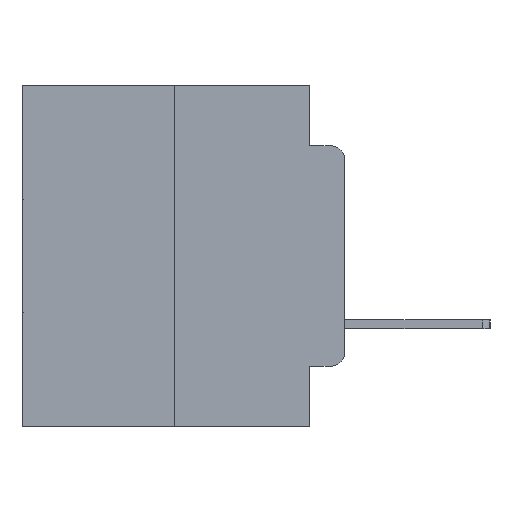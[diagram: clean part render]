
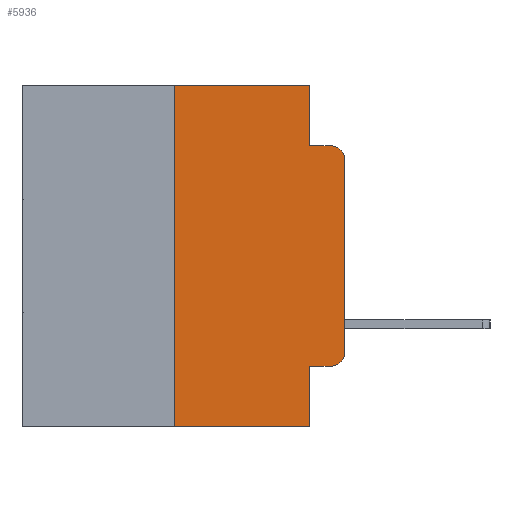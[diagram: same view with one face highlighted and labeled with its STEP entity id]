
A CAD part, left-side view. The second image highlights one B-rep face of the part: STEP entity #5936.
In plain terms, the highlighted planar face has unit normal (-1, 0, 0).
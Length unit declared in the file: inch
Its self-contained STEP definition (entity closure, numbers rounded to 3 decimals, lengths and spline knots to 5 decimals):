
#39 = DIRECTION ( 'NONE',  ( 0., -1., 0. ) ) ;
#232 = CARTESIAN_POINT ( 'NONE',  ( 0., 0.02, -0.4115 ) ) ;
#286 = VECTOR ( 'NONE', #25031, 39.37008 ) ;
#444 = EDGE_CURVE ( 'NONE', #7552, #21658, #17296, .T. ) ;
#829 = VERTEX_POINT ( 'NONE', #16610 ) ;
#1479 = DIRECTION ( 'NONE',  ( 0., -1., 0. ) ) ;
#1516 = ORIENTED_EDGE ( 'NONE', *, *, #5882, .T. ) ;
#1777 = LINE ( 'NONE', #26739, #12896 ) ;
#1890 = ORIENTED_EDGE ( 'NONE', *, *, #24686, .T. ) ;
#2066 = CARTESIAN_POINT ( 'NONE',  ( 0., 0.02, -0.3915 ) ) ;
#2331 = DIRECTION ( 'NONE',  ( 0., -1., 0. ) ) ;
#2914 = ORIENTED_EDGE ( 'NONE', *, *, #16534, .F. ) ;
#3414 = ORIENTED_EDGE ( 'NONE', *, *, #444, .F. ) ;
#3684 = ORIENTED_EDGE ( 'NONE', *, *, #9267, .F. ) ;
#3862 = AXIS2_PLACEMENT_3D ( 'NONE', #11210, #25497, #13319 ) ;
#3930 = ORIENTED_EDGE ( 'NONE', *, *, #17087, .F. ) ;
#3967 = EDGE_CURVE ( 'NONE', #19862, #829, #14197, .T. ) ;
#4100 = ORIENTED_EDGE ( 'NONE', *, *, #17632, .T. ) ;
#4322 = DIRECTION ( 'NONE',  ( 0., 0., -1. ) ) ;
#4430 = ORIENTED_EDGE ( 'NONE', *, *, #6991, .F. ) ;
#4480 = CARTESIAN_POINT ( 'NONE',  ( 0., 0.051, -0.5 ) ) ;
#4484 = ORIENTED_EDGE ( 'NONE', *, *, #5492, .T. ) ;
#4517 = VERTEX_POINT ( 'NONE', #4480 ) ;
#4648 = ORIENTED_EDGE ( 'NONE', *, *, #3967, .T. ) ;
#5492 = EDGE_CURVE ( 'NONE', #26529, #19862, #8429, .T. ) ;
#5882 = EDGE_CURVE ( 'NONE', #829, #21941, #13429, .T. ) ;
#5936 = ADVANCED_FACE ( 'NONE', ( #17036 ), #15282, .F. ) ;
#5951 = LINE ( 'NONE', #19071, #22824 ) ;
#6254 = DIRECTION ( 'NONE',  ( 0., 0., 1. ) ) ;
#6708 = CARTESIAN_POINT ( 'NONE',  ( 0., 0.25, -0.5 ) ) ;
#6991 = EDGE_CURVE ( 'NONE', #26529, #4517, #25455, .T. ) ;
#7493 = CARTESIAN_POINT ( 'NONE',  ( 0., 0.25, 0. ) ) ;
#7552 = VERTEX_POINT ( 'NONE', #13449 ) ;
#8314 = VECTOR ( 'NONE', #17233, 39.37008 ) ;
#8429 = LINE ( 'NONE', #15481, #24329 ) ;
#8680 = CIRCLE ( 'NONE', #3862, 0.02 ) ;
#9267 = EDGE_CURVE ( 'NONE', #25586, #7552, #17662, .T. ) ;
#10751 = CARTESIAN_POINT ( 'NONE',  ( 0., 0.051, -0.4115 ) ) ;
#10934 = CARTESIAN_POINT ( 'NONE',  ( 0., 0.051, 0. ) ) ;
#11016 = AXIS2_PLACEMENT_3D ( 'NONE', #2066, #17320, #4322 ) ;
#11167 = DIRECTION ( 'NONE',  ( 0., 0., -1. ) ) ;
#11210 = CARTESIAN_POINT ( 'NONE',  ( 0., 0.02, -0.1085 ) ) ;
#11452 = LINE ( 'NONE', #23502, #20583 ) ;
#12809 = VECTOR ( 'NONE', #15016, 39.37008 ) ;
#12842 = CARTESIAN_POINT ( 'NONE',  ( 0., 0.473, 0. ) ) ;
#12896 = VECTOR ( 'NONE', #1479, 39.37008 ) ;
#13020 = CARTESIAN_POINT ( 'NONE',  ( 0., 0., 0. ) ) ;
#13319 = DIRECTION ( 'NONE',  ( 0., 0., -1. ) ) ;
#13429 = LINE ( 'NONE', #13020, #12809 ) ;
#13449 = CARTESIAN_POINT ( 'NONE',  ( 0., 0.051, 0. ) ) ;
#14048 = DIRECTION ( 'NONE',  ( 0., 0., -1. ) ) ;
#14197 = CIRCLE ( 'NONE', #11016, 0.02 ) ;
#14690 = CARTESIAN_POINT ( 'NONE',  ( 0., 0.051, -0.0885 ) ) ;
#15016 = DIRECTION ( 'NONE',  ( 0., 0., 1. ) ) ;
#15102 = AXIS2_PLACEMENT_3D ( 'NONE', #19458, #23497, #11167 ) ;
#15282 = PLANE ( 'NONE',  #15102 ) ;
#15481 = CARTESIAN_POINT ( 'NONE',  ( 0., 0.051, -0.4115 ) ) ;
#15972 = VECTOR ( 'NONE', #14048, 39.37008 ) ;
#16534 = EDGE_CURVE ( 'NONE', #21658, #18693, #1777, .T. ) ;
#16610 = CARTESIAN_POINT ( 'NONE',  ( 0., 0., -0.3915 ) ) ;
#16893 = CARTESIAN_POINT ( 'NONE',  ( 0., 0.02, -0.0885 ) ) ;
#17036 = FACE_OUTER_BOUND ( 'NONE', #22107, .T. ) ;
#17087 = EDGE_CURVE ( 'NONE', #18920, #25586, #5951, .T. ) ;
#17233 = DIRECTION ( 'NONE',  ( 0., 0., -1. ) ) ;
#17296 = LINE ( 'NONE', #23672, #15972 ) ;
#17320 = DIRECTION ( 'NONE',  ( -1., 0., 0. ) ) ;
#17632 = EDGE_CURVE ( 'NONE', #18920, #4517, #11452, .T. ) ;
#17662 = LINE ( 'NONE', #12842, #286 ) ;
#18693 = VERTEX_POINT ( 'NONE', #16893 ) ;
#18920 = VERTEX_POINT ( 'NONE', #6708 ) ;
#19071 = CARTESIAN_POINT ( 'NONE',  ( 0., 0.25, 0. ) ) ;
#19458 = CARTESIAN_POINT ( 'NONE',  ( 0., 0.473, 0. ) ) ;
#19862 = VERTEX_POINT ( 'NONE', #232 ) ;
#20583 = VECTOR ( 'NONE', #39, 39.37008 ) ;
#21658 = VERTEX_POINT ( 'NONE', #14690 ) ;
#21941 = VERTEX_POINT ( 'NONE', #25573 ) ;
#22107 = EDGE_LOOP ( 'NONE', ( #1516, #1890, #2914, #3414, #3684, #3930, #4100, #4430, #4484, #4648 ) ) ;
#22824 = VECTOR ( 'NONE', #6254, 39.37008 ) ;
#23497 = DIRECTION ( 'NONE',  ( 1., 0., 0. ) ) ;
#23502 = CARTESIAN_POINT ( 'NONE',  ( 0., 0.473, -0.5 ) ) ;
#23672 = CARTESIAN_POINT ( 'NONE',  ( 0., 0.051, 0. ) ) ;
#24329 = VECTOR ( 'NONE', #2331, 39.37008 ) ;
#24686 = EDGE_CURVE ( 'NONE', #21941, #18693, #8680, .T. ) ;
#25031 = DIRECTION ( 'NONE',  ( 0., -1., 0. ) ) ;
#25455 = LINE ( 'NONE', #10934, #8314 ) ;
#25497 = DIRECTION ( 'NONE',  ( -1., 0., 0. ) ) ;
#25573 = CARTESIAN_POINT ( 'NONE',  ( 0., 0., -0.1085 ) ) ;
#25586 = VERTEX_POINT ( 'NONE', #7493 ) ;
#26529 = VERTEX_POINT ( 'NONE', #10751 ) ;
#26739 = CARTESIAN_POINT ( 'NONE',  ( 0., 0.051, -0.0885 ) ) ;
